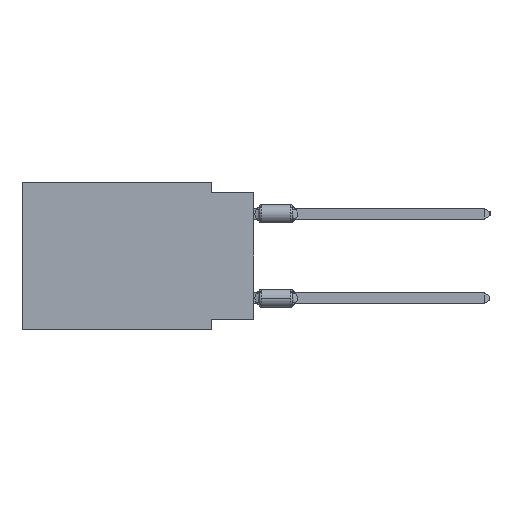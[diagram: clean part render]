
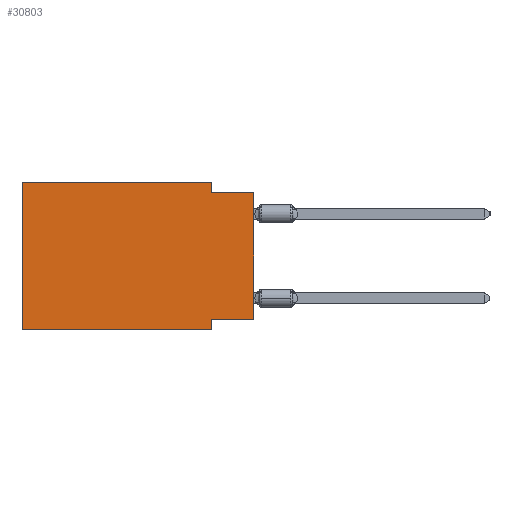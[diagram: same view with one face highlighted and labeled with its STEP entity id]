
A CAD part, left-side view. The second image highlights one B-rep face of the part: STEP entity #30803.
In plain terms, the highlighted planar face has unit normal (-1, 0, 0).
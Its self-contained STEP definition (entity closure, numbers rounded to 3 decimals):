
#269 = LINE ( 'NONE', #15406, #24496 ) ;
#2263 = DIRECTION ( 'NONE',  ( 0., -1., 0. ) ) ;
#2691 = LINE ( 'NONE', #7320, #23364 ) ;
#3021 = DIRECTION ( 'NONE',  ( 0., -1., 0. ) ) ;
#3864 = VERTEX_POINT ( 'NONE', #23765 ) ;
#4462 = ORIENTED_EDGE ( 'NONE', *, *, #27526, .F. ) ;
#4832 = CARTESIAN_POINT ( 'NONE',  ( 0., 0., -0.635 ) ) ;
#5224 = DIRECTION ( 'NONE',  ( 0., 0., 1. ) ) ;
#6078 = PLANE ( 'NONE',  #21509 ) ;
#6407 = CARTESIAN_POINT ( 'NONE',  ( 0., 13.97, 0. ) ) ;
#6894 = DIRECTION ( 'NONE',  ( 1., 0., 0. ) ) ;
#7053 = VERTEX_POINT ( 'NONE', #27381 ) ;
#7101 = VERTEX_POINT ( 'NONE', #24583 ) ;
#7281 = LINE ( 'NONE', #24690, #13524 ) ;
#7320 = CARTESIAN_POINT ( 'NONE',  ( 0., 0., 0. ) ) ;
#7688 = LINE ( 'NONE', #27738, #19190 ) ;
#8242 = DIRECTION ( 'NONE',  ( 0., 0., -1. ) ) ;
#9368 = ORIENTED_EDGE ( 'NONE', *, *, #29099, .F. ) ;
#9639 = EDGE_CURVE ( 'NONE', #19505, #31534, #269, .T. ) ;
#10423 = DIRECTION ( 'NONE',  ( 0., 0., 1. ) ) ;
#10983 = DIRECTION ( 'NONE',  ( 0., 0., -1. ) ) ;
#11128 = ORIENTED_EDGE ( 'NONE', *, *, #23833, .T. ) ;
#11659 = EDGE_CURVE ( 'NONE', #17079, #20615, #29397, .T. ) ;
#12420 = CARTESIAN_POINT ( 'NONE',  ( 0., 13.97, 0. ) ) ;
#12467 = CARTESIAN_POINT ( 'NONE',  ( 0., 0., -0.635 ) ) ;
#12874 = ORIENTED_EDGE ( 'NONE', *, *, #9639, .T. ) ;
#12967 = VERTEX_POINT ( 'NONE', #25742 ) ;
#13042 = ORIENTED_EDGE ( 'NONE', *, *, #31815, .F. ) ;
#13524 = VECTOR ( 'NONE', #25169, 1000. ) ;
#15406 = CARTESIAN_POINT ( 'NONE',  ( 0., 13.97, -8.89 ) ) ;
#16402 = ORIENTED_EDGE ( 'NONE', *, *, #32260, .F. ) ;
#16909 = DIRECTION ( 'NONE',  ( 0., 0., -1. ) ) ;
#17079 = VERTEX_POINT ( 'NONE', #21153 ) ;
#18269 = LINE ( 'NONE', #21046, #21575 ) ;
#19050 = ORIENTED_EDGE ( 'NONE', *, *, #11659, .F. ) ;
#19190 = VECTOR ( 'NONE', #5224, 1000. ) ;
#19505 = VERTEX_POINT ( 'NONE', #30965 ) ;
#20526 = CARTESIAN_POINT ( 'NONE',  ( 0., 2.54, 0. ) ) ;
#20614 = VECTOR ( 'NONE', #3021, 1000. ) ;
#20615 = VERTEX_POINT ( 'NONE', #4832 ) ;
#21046 = CARTESIAN_POINT ( 'NONE',  ( 0., 2.54, -8.89 ) ) ;
#21153 = CARTESIAN_POINT ( 'NONE',  ( 0., 2.54, -0.635 ) ) ;
#21509 = AXIS2_PLACEMENT_3D ( 'NONE', #6407, #6894, #16909 ) ;
#21575 = VECTOR ( 'NONE', #8242, 1000. ) ;
#22587 = LINE ( 'NONE', #12420, #20614 ) ;
#23142 = LINE ( 'NONE', #20526, #27715 ) ;
#23364 = VECTOR ( 'NONE', #10423, 1000. ) ;
#23765 = CARTESIAN_POINT ( 'NONE',  ( 0., 0., -8.255 ) ) ;
#23833 = EDGE_CURVE ( 'NONE', #3864, #20615, #2691, .T. ) ;
#24496 = VECTOR ( 'NONE', #30697, 1000. ) ;
#24583 = CARTESIAN_POINT ( 'NONE',  ( 0., 2.54, -8.255 ) ) ;
#24690 = CARTESIAN_POINT ( 'NONE',  ( 0., 0., -8.255 ) ) ;
#25035 = EDGE_CURVE ( 'NONE', #7053, #12967, #22587, .T. ) ;
#25169 = DIRECTION ( 'NONE',  ( 0., 1., 0. ) ) ;
#25385 = CARTESIAN_POINT ( 'NONE',  ( 0., 2.54, -8.89 ) ) ;
#25742 = CARTESIAN_POINT ( 'NONE',  ( 0., 2.54, 0. ) ) ;
#27381 = CARTESIAN_POINT ( 'NONE',  ( 0., 13.97, 0. ) ) ;
#27526 = EDGE_CURVE ( 'NONE', #19505, #7053, #7688, .T. ) ;
#27715 = VECTOR ( 'NONE', #10983, 1000. ) ;
#27738 = CARTESIAN_POINT ( 'NONE',  ( 0., 13.97, 0. ) ) ;
#28576 = FACE_OUTER_BOUND ( 'NONE', #28583, .T. ) ;
#28583 = EDGE_LOOP ( 'NONE', ( #11128, #19050, #16402, #32103, #4462, #12874, #9368, #13042 ) ) ;
#29099 = EDGE_CURVE ( 'NONE', #7101, #31534, #18269, .T. ) ;
#29282 = VECTOR ( 'NONE', #2263, 1000. ) ;
#29397 = LINE ( 'NONE', #12467, #29282 ) ;
#30697 = DIRECTION ( 'NONE',  ( 0., -1., 0. ) ) ;
#30803 = ADVANCED_FACE ( 'NONE', ( #28576 ), #6078, .F. ) ;
#30965 = CARTESIAN_POINT ( 'NONE',  ( 0., 13.97, -8.89 ) ) ;
#31534 = VERTEX_POINT ( 'NONE', #25385 ) ;
#31815 = EDGE_CURVE ( 'NONE', #3864, #7101, #7281, .T. ) ;
#32103 = ORIENTED_EDGE ( 'NONE', *, *, #25035, .F. ) ;
#32260 = EDGE_CURVE ( 'NONE', #12967, #17079, #23142, .T. ) ;
